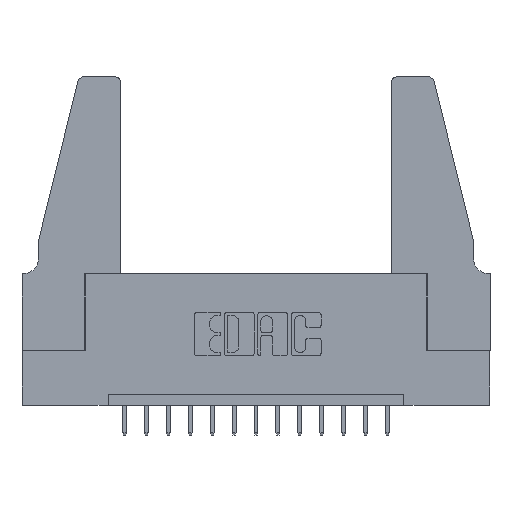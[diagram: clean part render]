
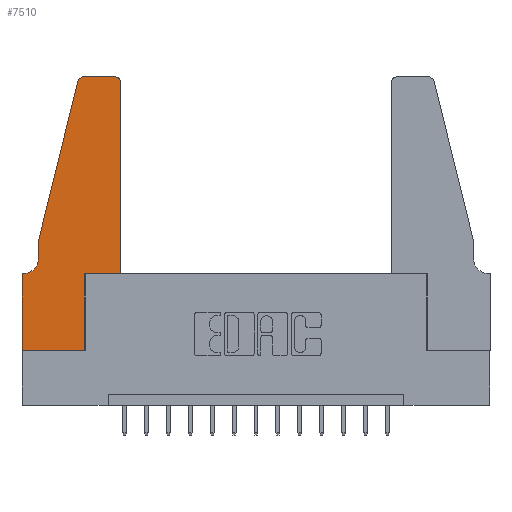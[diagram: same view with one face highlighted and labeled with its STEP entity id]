
A CAD part, top view. The second image highlights one B-rep face of the part: STEP entity #7510.
In plain terms, the highlighted planar face has unit normal (0, 0, 1).
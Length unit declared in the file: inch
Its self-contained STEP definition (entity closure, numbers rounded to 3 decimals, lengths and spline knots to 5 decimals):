
#108 = CARTESIAN_POINT ( 'NONE',  ( 0.0755, 0.5, 0.37 ) ) ;
#250 = LINE ( 'NONE', #11083, #7276 ) ;
#331 = AXIS2_PLACEMENT_3D ( 'NONE', #1949, #11999, #14348 ) ;
#456 = DIRECTION ( 'NONE',  ( -1., 0., 0. ) ) ;
#522 = CARTESIAN_POINT ( 'NONE',  ( 0.0055, 0.42, 0.37 ) ) ;
#710 = LINE ( 'NONE', #15460, #2393 ) ;
#967 = VERTEX_POINT ( 'NONE', #13792 ) ;
#1049 = DIRECTION ( 'NONE',  ( 1., 0., 0. ) ) ;
#1116 = EDGE_CURVE ( 'NONE', #14973, #8530, #10636, .T. ) ;
#1284 = CARTESIAN_POINT ( 'NONE',  ( 0., 0.35, 0.37 ) ) ;
#1713 = CARTESIAN_POINT ( 'NONE',  ( 0.4205, 1.22, 0.37 ) ) ;
#1810 = ORIENTED_EDGE ( 'NONE', *, *, #8378, .T. ) ;
#1949 = CARTESIAN_POINT ( 'NONE',  ( 0.284, 1.22, 0.37 ) ) ;
#2199 = CARTESIAN_POINT ( 'NONE',  ( 0.4505, 0.35, 0.37 ) ) ;
#2239 = EDGE_CURVE ( 'NONE', #14574, #14531, #250, .T. ) ;
#2393 = VECTOR ( 'NONE', #7208, 39.37008 ) ;
#2499 = DIRECTION ( 'NONE',  ( 0., -1., 0. ) ) ;
#2560 = CARTESIAN_POINT ( 'NONE',  ( 0.25487, 1.22718, 0.37 ) ) ;
#2635 = ORIENTED_EDGE ( 'NONE', *, *, #9828, .T. ) ;
#2737 = CARTESIAN_POINT ( 'NONE',  ( 0., 0.35, 0.37 ) ) ;
#2753 = DIRECTION ( 'NONE',  ( -1., 0., 0. ) ) ;
#2843 = CARTESIAN_POINT ( 'NONE',  ( 0.2605, 1.25, 0.37 ) ) ;
#3145 = DIRECTION ( 'NONE',  ( 1., 0., 0. ) ) ;
#3536 = EDGE_CURVE ( 'NONE', #4414, #13700, #15450, .T. ) ;
#3597 = CARTESIAN_POINT ( 'NONE',  ( 0.0755, 0.5, 0.37 ) ) ;
#4414 = VERTEX_POINT ( 'NONE', #7241 ) ;
#4439 = VERTEX_POINT ( 'NONE', #6029 ) ;
#4442 = CARTESIAN_POINT ( 'NONE',  ( 0., 0., 0.37 ) ) ;
#4509 = CIRCLE ( 'NONE', #15644, 0.07 ) ;
#4633 = EDGE_CURVE ( 'NONE', #7697, #4439, #4509, .T. ) ;
#4793 = ORIENTED_EDGE ( 'NONE', *, *, #3536, .T. ) ;
#5841 = CARTESIAN_POINT ( 'NONE',  ( 0.2865, 0.35, 0.37 ) ) ;
#5951 = CIRCLE ( 'NONE', #331, 0.03 ) ;
#6029 = CARTESIAN_POINT ( 'NONE',  ( 0.0055, 0.35, 0.37 ) ) ;
#6100 = ORIENTED_EDGE ( 'NONE', *, *, #10775, .T. ) ;
#6171 = ORIENTED_EDGE ( 'NONE', *, *, #7896, .T. ) ;
#6264 = LINE ( 'NONE', #108, #7552 ) ;
#6299 = DIRECTION ( 'NONE',  ( 0., 0., -1. ) ) ;
#6524 = VECTOR ( 'NONE', #11944, 39.37008 ) ;
#6598 = DIRECTION ( 'NONE',  ( 0., 1., 0. ) ) ;
#6759 = CARTESIAN_POINT ( 'NONE',  ( 0.4505, 0.35, 0.37 ) ) ;
#6763 = VECTOR ( 'NONE', #3145, 39.37008 ) ;
#6841 = CARTESIAN_POINT ( 'NONE',  ( 0.284, 1.25, 0.37 ) ) ;
#6909 = EDGE_CURVE ( 'NONE', #13700, #14574, #5951, .T. ) ;
#7208 = DIRECTION ( 'NONE',  ( -1., 0., 0. ) ) ;
#7241 = CARTESIAN_POINT ( 'NONE',  ( 0.4205, 1.25, 0.37 ) ) ;
#7276 = VECTOR ( 'NONE', #13598, 39.37008 ) ;
#7317 = VECTOR ( 'NONE', #15818, 39.37008 ) ;
#7437 = ORIENTED_EDGE ( 'NONE', *, *, #2239, .T. ) ;
#7485 = ORIENTED_EDGE ( 'NONE', *, *, #13760, .T. ) ;
#7510 = ADVANCED_FACE ( 'NONE', ( #8516 ), #12220, .T. ) ;
#7552 = VECTOR ( 'NONE', #2499, 39.37008 ) ;
#7697 = VERTEX_POINT ( 'NONE', #13746 ) ;
#7787 = VECTOR ( 'NONE', #456, 39.37008 ) ;
#7838 = CIRCLE ( 'NONE', #9661, 0.03 ) ;
#7896 = EDGE_CURVE ( 'NONE', #4439, #12359, #710, .T. ) ;
#7984 = DIRECTION ( 'NONE',  ( 1., 0., 0. ) ) ;
#8368 = ORIENTED_EDGE ( 'NONE', *, *, #4633, .T. ) ;
#8378 = EDGE_CURVE ( 'NONE', #14531, #7697, #6264, .T. ) ;
#8516 = FACE_OUTER_BOUND ( 'NONE', #10668, .T. ) ;
#8530 = VERTEX_POINT ( 'NONE', #12735 ) ;
#9445 = VECTOR ( 'NONE', #6598, 39.37008 ) ;
#9550 = EDGE_CURVE ( 'NONE', #12359, #15816, #9840, .T. ) ;
#9661 = AXIS2_PLACEMENT_3D ( 'NONE', #1713, #10300, #7984 ) ;
#9789 = ORIENTED_EDGE ( 'NONE', *, *, #9550, .T. ) ;
#9828 = EDGE_CURVE ( 'NONE', #967, #4414, #7838, .T. ) ;
#9840 = LINE ( 'NONE', #13561, #6524 ) ;
#10300 = DIRECTION ( 'NONE',  ( 0., 0., 1. ) ) ;
#10382 = CARTESIAN_POINT ( 'NONE',  ( 0., 0., 0.37 ) ) ;
#10636 = LINE ( 'NONE', #2199, #6763 ) ;
#10668 = EDGE_LOOP ( 'NONE', ( #4793, #11158, #7437, #1810, #8368, #6171, #9789, #6100, #15264, #14290, #7485, #2635 ) ) ;
#10775 = EDGE_CURVE ( 'NONE', #15816, #13726, #12935, .T. ) ;
#11083 = CARTESIAN_POINT ( 'NONE',  ( 0.0755, 0.5, 0.37 ) ) ;
#11158 = ORIENTED_EDGE ( 'NONE', *, *, #6909, .T. ) ;
#11313 = EDGE_CURVE ( 'NONE', #13726, #14973, #14571, .T. ) ;
#11685 = CARTESIAN_POINT ( 'NONE',  ( 0.2865, 0., 0.37 ) ) ;
#11944 = DIRECTION ( 'NONE',  ( 0., -1., 0. ) ) ;
#11999 = DIRECTION ( 'NONE',  ( 0., 0., 1. ) ) ;
#12220 = PLANE ( 'NONE',  #13454 ) ;
#12359 = VERTEX_POINT ( 'NONE', #2737 ) ;
#12735 = CARTESIAN_POINT ( 'NONE',  ( 0.4505, 0.35, 0.37 ) ) ;
#12935 = LINE ( 'NONE', #4442, #14011 ) ;
#13369 = DIRECTION ( 'NONE',  ( 0., 0., 1. ) ) ;
#13454 = AXIS2_PLACEMENT_3D ( 'NONE', #1284, #13369, #1049 ) ;
#13561 = CARTESIAN_POINT ( 'NONE',  ( 0., 0., 0.37 ) ) ;
#13598 = DIRECTION ( 'NONE',  ( -0.239, -0.971, 0. ) ) ;
#13700 = VERTEX_POINT ( 'NONE', #6841 ) ;
#13726 = VERTEX_POINT ( 'NONE', #11685 ) ;
#13746 = CARTESIAN_POINT ( 'NONE',  ( 0.0755, 0.42, 0.37 ) ) ;
#13760 = EDGE_CURVE ( 'NONE', #8530, #967, #14031, .T. ) ;
#13792 = CARTESIAN_POINT ( 'NONE',  ( 0.4505, 1.22, 0.37 ) ) ;
#13873 = CARTESIAN_POINT ( 'NONE',  ( 0.2865, 0.35, 0.37 ) ) ;
#14011 = VECTOR ( 'NONE', #15623, 39.37008 ) ;
#14031 = LINE ( 'NONE', #6759, #9445 ) ;
#14290 = ORIENTED_EDGE ( 'NONE', *, *, #1116, .T. ) ;
#14348 = DIRECTION ( 'NONE',  ( 1., 0., 0. ) ) ;
#14531 = VERTEX_POINT ( 'NONE', #3597 ) ;
#14571 = LINE ( 'NONE', #5841, #7317 ) ;
#14574 = VERTEX_POINT ( 'NONE', #2560 ) ;
#14973 = VERTEX_POINT ( 'NONE', #13873 ) ;
#15264 = ORIENTED_EDGE ( 'NONE', *, *, #11313, .T. ) ;
#15450 = LINE ( 'NONE', #2843, #7787 ) ;
#15460 = CARTESIAN_POINT ( 'NONE',  ( 0.0755, 0.35, 0.37 ) ) ;
#15623 = DIRECTION ( 'NONE',  ( 1., 0., 0. ) ) ;
#15644 = AXIS2_PLACEMENT_3D ( 'NONE', #522, #6299, #2753 ) ;
#15816 = VERTEX_POINT ( 'NONE', #10382 ) ;
#15818 = DIRECTION ( 'NONE',  ( 0., 1., 0. ) ) ;
